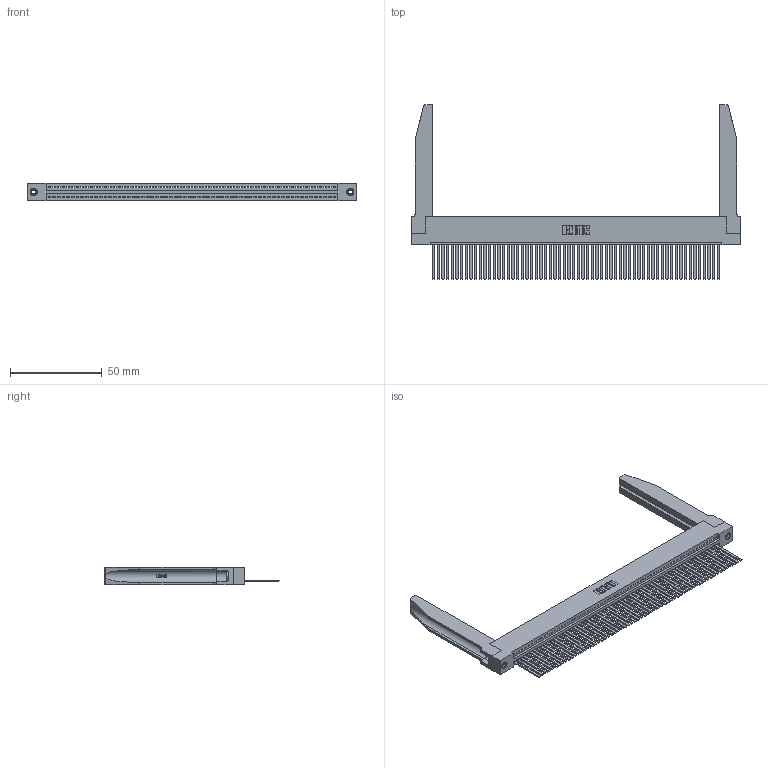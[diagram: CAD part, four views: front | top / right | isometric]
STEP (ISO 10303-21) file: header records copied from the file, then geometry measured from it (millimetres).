
FILE_DESCRIPTION (( 'STEP AP203' ), '1' );
FILE_NAME ('345-062-544-178.STEP', '2019-10-11T07:27:33', ( '' ), ( '' ), 'SwSTEP 2.0', 'SolidWorks 2016', '' );
FILE_SCHEMA (( 'CONFIG_CONTROL_DESIGN' ));
Length unit declared in the file: inch
Products named in the file (5): 345-220-078_345-220-078; 345-062-544-178; 345-250-001_345-250-001-102; 345 Part_Flush Mounting Lugs - 0.156 Dia-TH; 345-292-001_345-293-144
Assembly tree (67 placements, depth 2):
  345-062-544-178
    345 Part_Flush Mounting Lugs - 0.156 Dia-TH
    345-292-001_345-293-144  x62
    345-250-001_345-250-001-102  x2
    345-220-078_345-220-078  x2
Bounding box: 178.71 x 94.92 x 9.4 mm (x, y, z)
Volume: 25626.8 mm3; surface area: 33002.5 mm2
Topology: 67 solids, 67 shells, 3584 faces, 10745 edges, 7070 vertices
Faces by surface type: plane 2454, cylinder 1078, bspline 36, cone 12, torus 4
Entity records: 48526 total; most frequent: CARTESIAN_POINT 9301, ORIENTED_EDGE 8194, DIRECTION 7099, EDGE_CURVE 4097, VECTOR 3627, LINE 3627, VERTEX_POINT 2724, AXIS2_PLACEMENT_3D 1736
